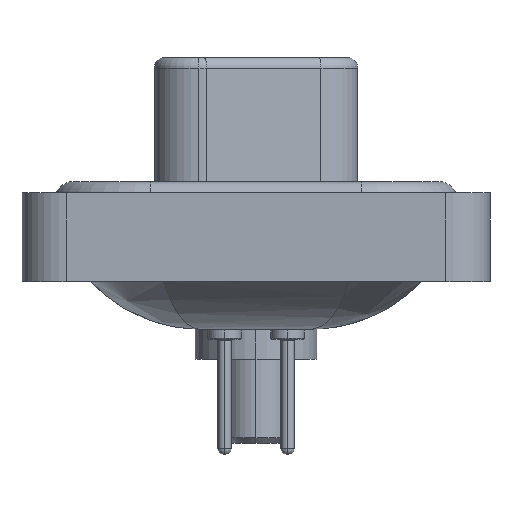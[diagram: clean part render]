
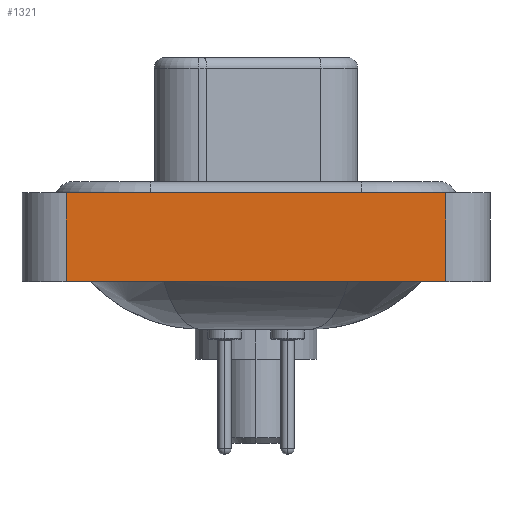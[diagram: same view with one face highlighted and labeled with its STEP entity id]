
A CAD part, left-side view. The second image highlights one B-rep face of the part: STEP entity #1321.
In plain terms, the highlighted planar face has unit normal (-1, 0, 0).
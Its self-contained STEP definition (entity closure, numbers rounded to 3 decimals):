
#271 = LINE ( 'NONE', #19170, #1096 ) ;
#1096 = VECTOR ( 'NONE', #9685, 1000. ) ;
#1321 = ADVANCED_FACE ( 'NONE', ( #14151 ), #6532, .T. ) ;
#2324 = EDGE_CURVE ( 'NONE', #13535, #3292, #271, .T. ) ;
#2796 = EDGE_CURVE ( 'NONE', #13535, #7289, #5066, .T. ) ;
#3114 = LINE ( 'NONE', #19090, #5283 ) ;
#3292 = VERTEX_POINT ( 'NONE', #19854 ) ;
#3300 = DIRECTION ( 'NONE',  ( 0., 0., 1. ) ) ;
#3591 = CARTESIAN_POINT ( 'NONE',  ( -7.3, 8.55, -3.6 ) ) ;
#4493 = ORIENTED_EDGE ( 'NONE', *, *, #20612, .F. ) ;
#5016 = CARTESIAN_POINT ( 'NONE',  ( -7.3, 8.55, -3.6 ) ) ;
#5023 = VECTOR ( 'NONE', #7405, 1000. ) ;
#5066 = LINE ( 'NONE', #3591, #5481 ) ;
#5283 = VECTOR ( 'NONE', #11451, 1000. ) ;
#5481 = VECTOR ( 'NONE', #9770, 1000. ) ;
#6523 = ORIENTED_EDGE ( 'NONE', *, *, #2324, .T. ) ;
#6532 = PLANE ( 'NONE',  #15313 ) ;
#7289 = VERTEX_POINT ( 'NONE', #15262 ) ;
#7405 = DIRECTION ( 'NONE',  ( 0., -1., 0. ) ) ;
#7702 = LINE ( 'NONE', #15302, #5023 ) ;
#9685 = DIRECTION ( 'NONE',  ( 0., -1., 0. ) ) ;
#9770 = DIRECTION ( 'NONE',  ( 0., 0., 1. ) ) ;
#10142 = ORIENTED_EDGE ( 'NONE', *, *, #2796, .F. ) ;
#10580 = EDGE_LOOP ( 'NONE', ( #12108, #4493, #10142, #6523 ) ) ;
#11233 = CARTESIAN_POINT ( 'NONE',  ( -7.3, -8.55, -3.6 ) ) ;
#11451 = DIRECTION ( 'NONE',  ( 0., 0., 1. ) ) ;
#12091 = VERTEX_POINT ( 'NONE', #19547 ) ;
#12108 = ORIENTED_EDGE ( 'NONE', *, *, #20270, .T. ) ;
#13535 = VERTEX_POINT ( 'NONE', #5016 ) ;
#14151 = FACE_OUTER_BOUND ( 'NONE', #10580, .T. ) ;
#15262 = CARTESIAN_POINT ( 'NONE',  ( -7.3, 8.55, 0.4 ) ) ;
#15302 = CARTESIAN_POINT ( 'NONE',  ( -7.3, -8.55, 0.4 ) ) ;
#15313 = AXIS2_PLACEMENT_3D ( 'NONE', #11233, #18963, #3300 ) ;
#18963 = DIRECTION ( 'NONE',  ( -1., 0., 0. ) ) ;
#19090 = CARTESIAN_POINT ( 'NONE',  ( -7.3, -8.55, -3.6 ) ) ;
#19170 = CARTESIAN_POINT ( 'NONE',  ( -7.3, -8.55, -3.6 ) ) ;
#19547 = CARTESIAN_POINT ( 'NONE',  ( -7.3, -8.55, 0.4 ) ) ;
#19854 = CARTESIAN_POINT ( 'NONE',  ( -7.3, -8.55, -3.6 ) ) ;
#20270 = EDGE_CURVE ( 'NONE', #3292, #12091, #3114, .T. ) ;
#20612 = EDGE_CURVE ( 'NONE', #7289, #12091, #7702, .T. ) ;
